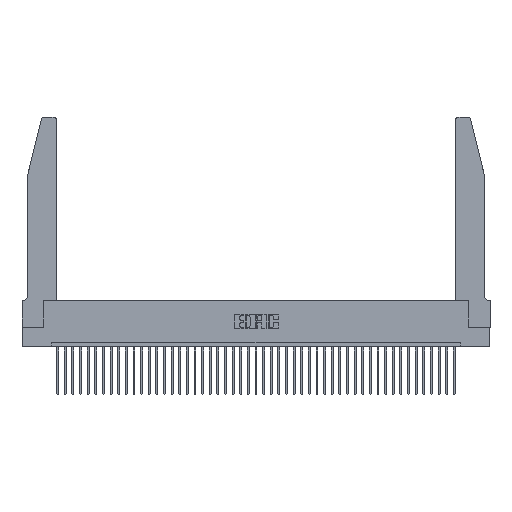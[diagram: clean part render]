
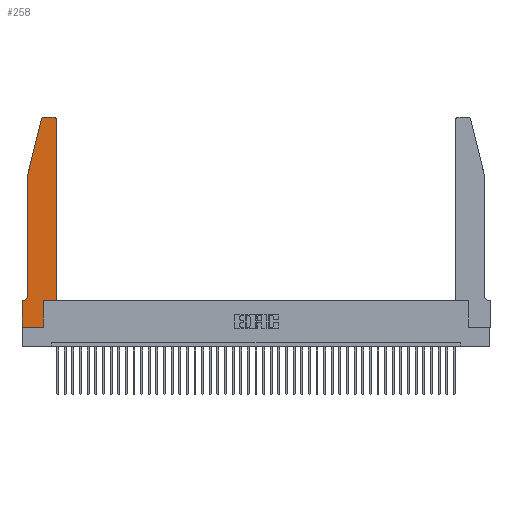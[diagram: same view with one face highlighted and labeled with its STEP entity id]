
A CAD part, top view. The second image highlights one B-rep face of the part: STEP entity #258.
In plain terms, the highlighted planar face has unit normal (0, 0, 1).
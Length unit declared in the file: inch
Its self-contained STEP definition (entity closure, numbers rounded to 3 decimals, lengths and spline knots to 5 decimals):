
#258 = ADVANCED_FACE ( 'NONE', ( #23795 ), #31820, .T. ) ;
#712 = VECTOR ( 'NONE', #19312, 39.37008 ) ;
#849 = VECTOR ( 'NONE', #38705, 39.37008 ) ;
#885 = CIRCLE ( 'NONE', #34693, 0.03 ) ;
#1545 = AXIS2_PLACEMENT_3D ( 'NONE', #20747, #34565, #7437 ) ;
#1623 = CARTESIAN_POINT ( 'NONE',  ( 0.4505, 0.35, 0.37 ) ) ;
#1876 = LINE ( 'NONE', #22303, #849 ) ;
#2553 = CARTESIAN_POINT ( 'NONE',  ( 0.0055, 0.35, 0.37 ) ) ;
#2562 = CARTESIAN_POINT ( 'NONE',  ( 0.25487, 2.72718, 0.37 ) ) ;
#4482 = VERTEX_POINT ( 'NONE', #11444 ) ;
#4874 = LINE ( 'NONE', #5707, #712 ) ;
#5299 = VERTEX_POINT ( 'NONE', #35749 ) ;
#5650 = VERTEX_POINT ( 'NONE', #2562 ) ;
#5707 = CARTESIAN_POINT ( 'NONE',  ( 0.0755, 0.35, 0.37 ) ) ;
#5951 = EDGE_CURVE ( 'NONE', #14878, #9092, #42491, .T. ) ;
#5966 = CARTESIAN_POINT ( 'NONE',  ( 0.2605, 2.75, 0.37 ) ) ;
#6398 = DIRECTION ( 'NONE',  ( 0., 0., -1. ) ) ;
#6456 = ORIENTED_EDGE ( 'NONE', *, *, #39888, .T. ) ;
#7437 = DIRECTION ( 'NONE',  ( 1., 0., 0. ) ) ;
#8049 = DIRECTION ( 'NONE',  ( 1., 0., 0. ) ) ;
#8194 = EDGE_CURVE ( 'NONE', #9092, #29494, #22569, .T. ) ;
#8482 = CARTESIAN_POINT ( 'NONE',  ( 0.0755, 2., 0.37 ) ) ;
#8841 = CARTESIAN_POINT ( 'NONE',  ( 0., 0., 0.37 ) ) ;
#9092 = VERTEX_POINT ( 'NONE', #39754 ) ;
#9216 = ORIENTED_EDGE ( 'NONE', *, *, #40217, .T. ) ;
#9622 = LINE ( 'NONE', #5966, #38816 ) ;
#9816 = ORIENTED_EDGE ( 'NONE', *, *, #41219, .T. ) ;
#10009 = VECTOR ( 'NONE', #37538, 39.37008 ) ;
#10015 = VECTOR ( 'NONE', #34351, 39.37008 ) ;
#10236 = ORIENTED_EDGE ( 'NONE', *, *, #8194, .T. ) ;
#10769 = EDGE_CURVE ( 'NONE', #25354, #36508, #39518, .T. ) ;
#11284 = CARTESIAN_POINT ( 'NONE',  ( 0., 0.35, 0.37 ) ) ;
#11444 = CARTESIAN_POINT ( 'NONE',  ( 0., 0., 0.37 ) ) ;
#13154 = DIRECTION ( 'NONE',  ( -1., 0., 0. ) ) ;
#13585 = CARTESIAN_POINT ( 'NONE',  ( 0.0055, 0.42, 0.37 ) ) ;
#13841 = DIRECTION ( 'NONE',  ( 1., 0., 0. ) ) ;
#14569 = ORIENTED_EDGE ( 'NONE', *, *, #24468, .T. ) ;
#14878 = VERTEX_POINT ( 'NONE', #34147 ) ;
#15978 = CARTESIAN_POINT ( 'NONE',  ( 0.284, 2.75, 0.37 ) ) ;
#16271 = EDGE_CURVE ( 'NONE', #5299, #25354, #23160, .T. ) ;
#17182 = ORIENTED_EDGE ( 'NONE', *, *, #10769, .T. ) ;
#17200 = EDGE_LOOP ( 'NONE', ( #22604, #30801, #29193, #18693, #17182, #9816, #14569, #23474, #9216, #42687, #10236, #6456 ) ) ;
#18693 = ORIENTED_EDGE ( 'NONE', *, *, #16271, .T. ) ;
#19312 = DIRECTION ( 'NONE',  ( -1., 0., 0. ) ) ;
#19968 = DIRECTION ( 'NONE',  ( 0., 0., 1. ) ) ;
#20680 = VERTEX_POINT ( 'NONE', #21412 ) ;
#20747 = CARTESIAN_POINT ( 'NONE',  ( 0.284, 2.72, 0.37 ) ) ;
#20890 = CARTESIAN_POINT ( 'NONE',  ( 0.0755, 0.42, 0.37 ) ) ;
#21362 = DIRECTION ( 'NONE',  ( 1., 0., 0. ) ) ;
#21412 = CARTESIAN_POINT ( 'NONE',  ( 0.2865, 0., 0.37 ) ) ;
#21550 = CARTESIAN_POINT ( 'NONE',  ( 0.4505, 2.72, 0.37 ) ) ;
#22141 = CARTESIAN_POINT ( 'NONE',  ( 0., 0., 0.37 ) ) ;
#22303 = CARTESIAN_POINT ( 'NONE',  ( 0.2865, 0.35, 0.37 ) ) ;
#22438 = DIRECTION ( 'NONE',  ( 1., 0., 0. ) ) ;
#22569 = LINE ( 'NONE', #31020, #10015 ) ;
#22604 = ORIENTED_EDGE ( 'NONE', *, *, #29469, .T. ) ;
#23160 = LINE ( 'NONE', #8482, #29940 ) ;
#23382 = DIRECTION ( 'NONE',  ( -1., 0., 0. ) ) ;
#23474 = ORIENTED_EDGE ( 'NONE', *, *, #36375, .T. ) ;
#23795 = FACE_OUTER_BOUND ( 'NONE', #17200, .T. ) ;
#24216 = EDGE_CURVE ( 'NONE', #5650, #5299, #30893, .T. ) ;
#24468 = EDGE_CURVE ( 'NONE', #39224, #4482, #39203, .T. ) ;
#25081 = VERTEX_POINT ( 'NONE', #41414 ) ;
#25354 = VERTEX_POINT ( 'NONE', #20890 ) ;
#25783 = VECTOR ( 'NONE', #22438, 39.37008 ) ;
#25900 = AXIS2_PLACEMENT_3D ( 'NONE', #13585, #6398, #23382 ) ;
#27295 = CIRCLE ( 'NONE', #1545, 0.03 ) ;
#29193 = ORIENTED_EDGE ( 'NONE', *, *, #24216, .T. ) ;
#29469 = EDGE_CURVE ( 'NONE', #25081, #36468, #9622, .T. ) ;
#29494 = VERTEX_POINT ( 'NONE', #21550 ) ;
#29940 = VECTOR ( 'NONE', #41318, 39.37008 ) ;
#30045 = VECTOR ( 'NONE', #21362, 39.37008 ) ;
#30482 = CARTESIAN_POINT ( 'NONE',  ( 0.4205, 2.72, 0.37 ) ) ;
#30679 = EDGE_CURVE ( 'NONE', #36468, #5650, #27295, .T. ) ;
#30801 = ORIENTED_EDGE ( 'NONE', *, *, #30679, .T. ) ;
#30893 = LINE ( 'NONE', #40619, #10009 ) ;
#31020 = CARTESIAN_POINT ( 'NONE',  ( 0.4505, 0.35, 0.37 ) ) ;
#31820 = PLANE ( 'NONE',  #40092 ) ;
#32173 = DIRECTION ( 'NONE',  ( 0., -1., 0. ) ) ;
#34147 = CARTESIAN_POINT ( 'NONE',  ( 0.2865, 0.35, 0.37 ) ) ;
#34351 = DIRECTION ( 'NONE',  ( 0., 1., 0. ) ) ;
#34565 = DIRECTION ( 'NONE',  ( 0., 0., 1. ) ) ;
#34693 = AXIS2_PLACEMENT_3D ( 'NONE', #30482, #19968, #13841 ) ;
#35008 = VECTOR ( 'NONE', #32173, 39.37008 ) ;
#35749 = CARTESIAN_POINT ( 'NONE',  ( 0.0755, 2., 0.37 ) ) ;
#36375 = EDGE_CURVE ( 'NONE', #4482, #20680, #40325, .T. ) ;
#36468 = VERTEX_POINT ( 'NONE', #15978 ) ;
#36508 = VERTEX_POINT ( 'NONE', #2553 ) ;
#37538 = DIRECTION ( 'NONE',  ( -0.239, -0.971, 0. ) ) ;
#38500 = CARTESIAN_POINT ( 'NONE',  ( 0., 0.35, 0.37 ) ) ;
#38705 = DIRECTION ( 'NONE',  ( 0., 1., 0. ) ) ;
#38816 = VECTOR ( 'NONE', #13154, 39.37008 ) ;
#39203 = LINE ( 'NONE', #8841, #35008 ) ;
#39224 = VERTEX_POINT ( 'NONE', #38500 ) ;
#39518 = CIRCLE ( 'NONE', #25900, 0.07 ) ;
#39754 = CARTESIAN_POINT ( 'NONE',  ( 0.4505, 0.35, 0.37 ) ) ;
#39888 = EDGE_CURVE ( 'NONE', #29494, #25081, #885, .T. ) ;
#40092 = AXIS2_PLACEMENT_3D ( 'NONE', #11284, #41466, #8049 ) ;
#40217 = EDGE_CURVE ( 'NONE', #20680, #14878, #1876, .T. ) ;
#40325 = LINE ( 'NONE', #22141, #25783 ) ;
#40619 = CARTESIAN_POINT ( 'NONE',  ( 0.0755, 2., 0.37 ) ) ;
#41219 = EDGE_CURVE ( 'NONE', #36508, #39224, #4874, .T. ) ;
#41318 = DIRECTION ( 'NONE',  ( 0., -1., 0. ) ) ;
#41414 = CARTESIAN_POINT ( 'NONE',  ( 0.4205, 2.75, 0.37 ) ) ;
#41466 = DIRECTION ( 'NONE',  ( 0., 0., 1. ) ) ;
#42491 = LINE ( 'NONE', #1623, #30045 ) ;
#42687 = ORIENTED_EDGE ( 'NONE', *, *, #5951, .T. ) ;
